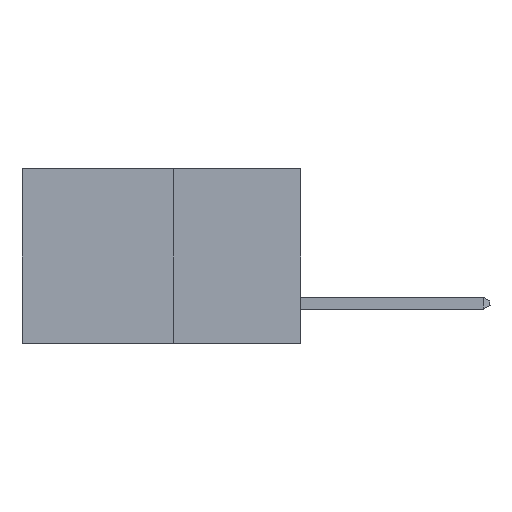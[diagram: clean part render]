
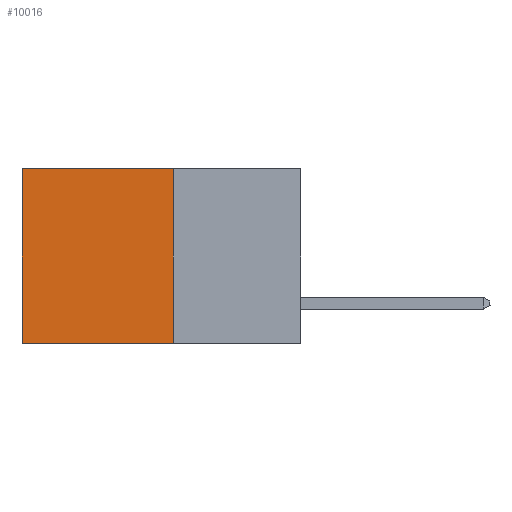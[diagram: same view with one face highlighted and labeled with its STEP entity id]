
A CAD part, left-side view. The second image highlights one B-rep face of the part: STEP entity #10016.
In plain terms, the highlighted planar face has unit normal (-1, 0, 0).
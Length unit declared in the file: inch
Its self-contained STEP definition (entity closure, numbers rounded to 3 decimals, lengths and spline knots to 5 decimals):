
#30 = CARTESIAN_POINT ( 'NONE',  ( 0.277, 0.59, 0. ) ) ;
#530 = DIRECTION ( 'NONE',  ( 1., 0., 0. ) ) ;
#734 = EDGE_CURVE ( 'NONE', #8425, #1034, #2503, .T. ) ;
#1034 = VERTEX_POINT ( 'NONE', #30 ) ;
#1760 = DIRECTION ( 'NONE',  ( 0., 1., 0. ) ) ;
#1859 = VECTOR ( 'NONE', #1760, 39.37008 ) ;
#2141 = VECTOR ( 'NONE', #10601, 39.37008 ) ;
#2197 = CARTESIAN_POINT ( 'NONE',  ( 0.277, 0.59, -0.37 ) ) ;
#2503 = LINE ( 'NONE', #6649, #1859 ) ;
#3385 = FACE_OUTER_BOUND ( 'NONE', #11831, .T. ) ;
#4539 = EDGE_CURVE ( 'NONE', #1034, #6811, #7060, .T. ) ;
#4886 = LINE ( 'NONE', #6494, #2141 ) ;
#5049 = ORIENTED_EDGE ( 'NONE', *, *, #734, .T. ) ;
#5175 = CARTESIAN_POINT ( 'NONE',  ( 0.277, 0.27, -0.37 ) ) ;
#5854 = CARTESIAN_POINT ( 'NONE',  ( 0.277, 0.27, 0. ) ) ;
#6188 = DIRECTION ( 'NONE',  ( 0., 0., -1. ) ) ;
#6494 = CARTESIAN_POINT ( 'NONE',  ( 0.277, 0.27, -0.37 ) ) ;
#6649 = CARTESIAN_POINT ( 'NONE',  ( 0.277, 0.27, 0. ) ) ;
#6811 = VERTEX_POINT ( 'NONE', #2197 ) ;
#6943 = ORIENTED_EDGE ( 'NONE', *, *, #7505, .F. ) ;
#7060 = LINE ( 'NONE', #8653, #12439 ) ;
#7401 = VERTEX_POINT ( 'NONE', #9406 ) ;
#7416 = ORIENTED_EDGE ( 'NONE', *, *, #4539, .T. ) ;
#7505 = EDGE_CURVE ( 'NONE', #7401, #6811, #4886, .T. ) ;
#7785 = DIRECTION ( 'NONE',  ( 0., 0., -1. ) ) ;
#8425 = VERTEX_POINT ( 'NONE', #5854 ) ;
#8653 = CARTESIAN_POINT ( 'NONE',  ( 0.277, 0.59, -0.37 ) ) ;
#8875 = DIRECTION ( 'NONE',  ( 0., 0., -1. ) ) ;
#9224 = ORIENTED_EDGE ( 'NONE', *, *, #12001, .F. ) ;
#9406 = CARTESIAN_POINT ( 'NONE',  ( 0.277, 0.27, -0.37 ) ) ;
#9802 = CARTESIAN_POINT ( 'NONE',  ( 0.277, 0.27, -0.37 ) ) ;
#10016 = ADVANCED_FACE ( 'NONE', ( #3385 ), #12815, .F. ) ;
#10554 = VECTOR ( 'NONE', #6188, 39.37008 ) ;
#10601 = DIRECTION ( 'NONE',  ( 0., 1., 0. ) ) ;
#10875 = LINE ( 'NONE', #5175, #10554 ) ;
#11831 = EDGE_LOOP ( 'NONE', ( #7416, #6943, #9224, #5049 ) ) ;
#11975 = AXIS2_PLACEMENT_3D ( 'NONE', #9802, #530, #7785 ) ;
#12001 = EDGE_CURVE ( 'NONE', #8425, #7401, #10875, .T. ) ;
#12439 = VECTOR ( 'NONE', #8875, 39.37008 ) ;
#12815 = PLANE ( 'NONE',  #11975 ) ;
